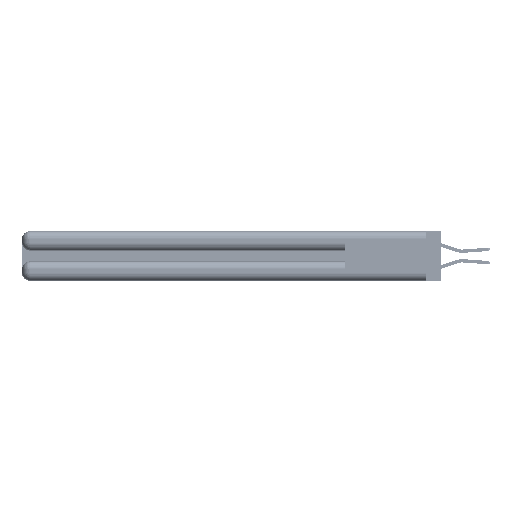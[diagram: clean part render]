
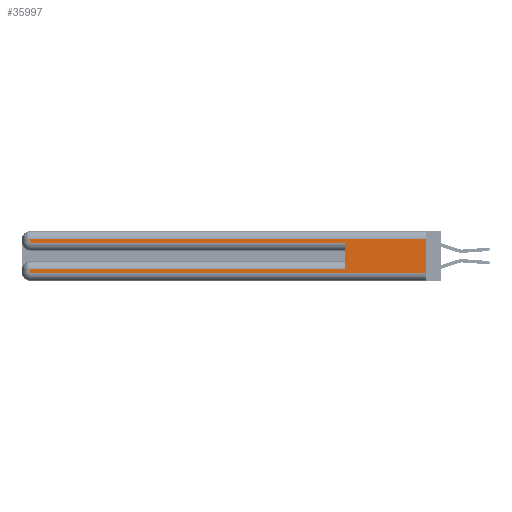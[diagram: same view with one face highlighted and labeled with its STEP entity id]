
A CAD part, left-side view. The second image highlights one B-rep face of the part: STEP entity #35997.
In plain terms, the highlighted planar face has unit normal (-1, 0, 0).
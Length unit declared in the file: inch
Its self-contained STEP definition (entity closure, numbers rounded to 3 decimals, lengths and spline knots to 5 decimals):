
#36 = DIRECTION ( 'NONE',  ( 0., -1., 0. ) ) ;
#2014 = CARTESIAN_POINT ( 'NONE',  ( 0., 2.94, 0.285 ) ) ;
#2276 = EDGE_CURVE ( 'NONE', #46327, #42064, #10809, .T. ) ;
#3293 = PLANE ( 'NONE',  #16571 ) ;
#3647 = VECTOR ( 'NONE', #11431, 39.37008 ) ;
#4652 = ORIENTED_EDGE ( 'NONE', *, *, #36158, .T. ) ;
#5285 = ORIENTED_EDGE ( 'NONE', *, *, #20421, .F. ) ;
#7247 = CARTESIAN_POINT ( 'NONE',  ( 0., 0., 0.285 ) ) ;
#7666 = CARTESIAN_POINT ( 'NONE',  ( 0., 2.94, 0.31 ) ) ;
#8563 = ORIENTED_EDGE ( 'NONE', *, *, #2276, .T. ) ;
#8956 = VERTEX_POINT ( 'NONE', #2014 ) ;
#9195 = ORIENTED_EDGE ( 'NONE', *, *, #49463, .T. ) ;
#10809 = LINE ( 'NONE', #16983, #13455 ) ;
#11431 = DIRECTION ( 'NONE',  ( 0., -1., 0. ) ) ;
#12774 = VERTEX_POINT ( 'NONE', #26482 ) ;
#13455 = VECTOR ( 'NONE', #46149, 39.37008 ) ;
#15848 = LINE ( 'NONE', #41940, #47786 ) ;
#15885 = CARTESIAN_POINT ( 'NONE',  ( 0., 0., 0.37 ) ) ;
#16044 = LINE ( 'NONE', #7247, #3647 ) ;
#16571 = AXIS2_PLACEMENT_3D ( 'NONE', #15885, #45025, #20037 ) ;
#16795 = CARTESIAN_POINT ( 'NONE',  ( 0., 2.94, 0.37 ) ) ;
#16983 = CARTESIAN_POINT ( 'NONE',  ( 0., 2.94, 0.37 ) ) ;
#18186 = VERTEX_POINT ( 'NONE', #46770 ) ;
#19994 = LINE ( 'NONE', #51908, #31078 ) ;
#20037 = DIRECTION ( 'NONE',  ( 0., 0., -1. ) ) ;
#20421 = EDGE_CURVE ( 'NONE', #18186, #29852, #36939, .T. ) ;
#20971 = DIRECTION ( 'NONE',  ( 0., 0., -1. ) ) ;
#23667 = FACE_OUTER_BOUND ( 'NONE', #40940, .T. ) ;
#25059 = CARTESIAN_POINT ( 'NONE',  ( 0., 0., 0.06 ) ) ;
#26482 = CARTESIAN_POINT ( 'NONE',  ( 0., 0.6, 0.085 ) ) ;
#26983 = DIRECTION ( 'NONE',  ( 0., 1., 0. ) ) ;
#27133 = VECTOR ( 'NONE', #29406, 39.37008 ) ;
#27842 = EDGE_CURVE ( 'NONE', #8956, #43066, #16044, .T. ) ;
#29165 = VERTEX_POINT ( 'NONE', #7666 ) ;
#29406 = DIRECTION ( 'NONE',  ( 0., 0., -1. ) ) ;
#29852 = VERTEX_POINT ( 'NONE', #42907 ) ;
#31078 = VECTOR ( 'NONE', #26983, 39.37008 ) ;
#32173 = CARTESIAN_POINT ( 'NONE',  ( 0., 2.94, 0.06 ) ) ;
#33749 = EDGE_CURVE ( 'NONE', #18186, #29165, #19994, .T. ) ;
#34773 = EDGE_CURVE ( 'NONE', #42064, #29852, #47937, .T. ) ;
#35791 = CARTESIAN_POINT ( 'NONE',  ( 0., 0.6, 0.145 ) ) ;
#35997 = ADVANCED_FACE ( 'NONE', ( #23667 ), #3293, .F. ) ;
#36158 = EDGE_CURVE ( 'NONE', #12774, #46327, #15848, .T. ) ;
#36939 = LINE ( 'NONE', #50136, #27133 ) ;
#39468 = CARTESIAN_POINT ( 'NONE',  ( 0., 2.94, 0.085 ) ) ;
#40008 = DIRECTION ( 'NONE',  ( 0., 0., 1. ) ) ;
#40940 = EDGE_LOOP ( 'NONE', ( #5285, #49572, #9195, #42482, #46387, #4652, #8563, #52825 ) ) ;
#41940 = CARTESIAN_POINT ( 'NONE',  ( 0., 0., 0.085 ) ) ;
#42064 = VERTEX_POINT ( 'NONE', #32173 ) ;
#42482 = ORIENTED_EDGE ( 'NONE', *, *, #27842, .T. ) ;
#42510 = LINE ( 'NONE', #35791, #52188 ) ;
#42907 = CARTESIAN_POINT ( 'NONE',  ( 0., 0., 0.06 ) ) ;
#43066 = VERTEX_POINT ( 'NONE', #48841 ) ;
#44724 = VECTOR ( 'NONE', #20971, 39.37008 ) ;
#45025 = DIRECTION ( 'NONE',  ( 1., 0., 0. ) ) ;
#46105 = DIRECTION ( 'NONE',  ( 0., 1., 0. ) ) ;
#46149 = DIRECTION ( 'NONE',  ( 0., 0., -1. ) ) ;
#46327 = VERTEX_POINT ( 'NONE', #39468 ) ;
#46387 = ORIENTED_EDGE ( 'NONE', *, *, #46392, .F. ) ;
#46392 = EDGE_CURVE ( 'NONE', #12774, #43066, #42510, .T. ) ;
#46770 = CARTESIAN_POINT ( 'NONE',  ( 0., 0., 0.31 ) ) ;
#47351 = LINE ( 'NONE', #16795, #44724 ) ;
#47786 = VECTOR ( 'NONE', #46105, 39.37008 ) ;
#47937 = LINE ( 'NONE', #25059, #49228 ) ;
#48841 = CARTESIAN_POINT ( 'NONE',  ( 0., 0.6, 0.285 ) ) ;
#49228 = VECTOR ( 'NONE', #36, 39.37008 ) ;
#49463 = EDGE_CURVE ( 'NONE', #29165, #8956, #47351, .T. ) ;
#49572 = ORIENTED_EDGE ( 'NONE', *, *, #33749, .T. ) ;
#50136 = CARTESIAN_POINT ( 'NONE',  ( 0., 0., 0.37 ) ) ;
#51908 = CARTESIAN_POINT ( 'NONE',  ( 0., 0., 0.31 ) ) ;
#52188 = VECTOR ( 'NONE', #40008, 39.37008 ) ;
#52825 = ORIENTED_EDGE ( 'NONE', *, *, #34773, .T. ) ;
